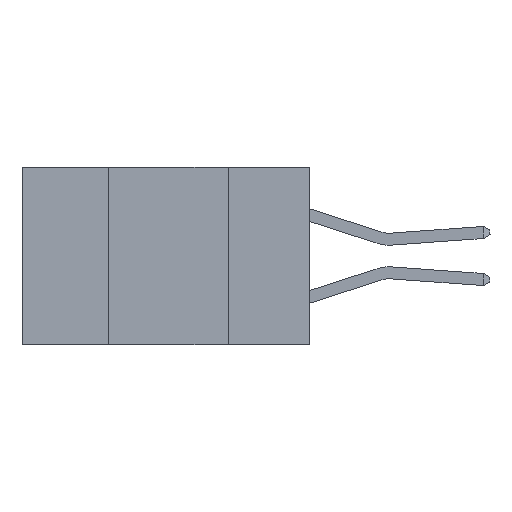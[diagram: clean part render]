
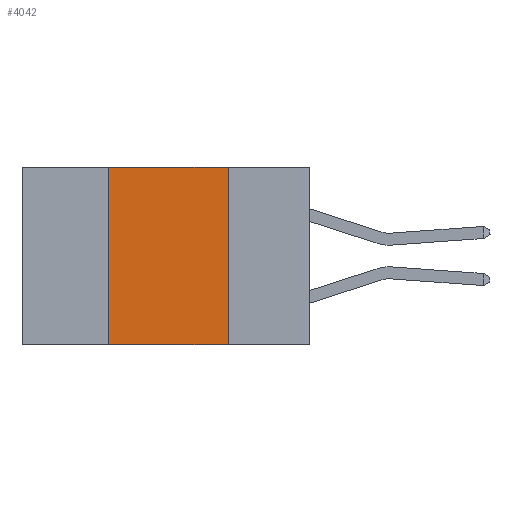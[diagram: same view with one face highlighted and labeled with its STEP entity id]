
A CAD part, left-side view. The second image highlights one B-rep face of the part: STEP entity #4042.
In plain terms, the highlighted planar face has unit normal (-1, 0, 0).
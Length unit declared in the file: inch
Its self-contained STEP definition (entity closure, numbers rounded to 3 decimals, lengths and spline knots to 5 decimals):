
#372 = EDGE_CURVE ( 'NONE', #27670, #22646, #2584, .T. ) ;
#1957 = EDGE_LOOP ( 'NONE', ( #6689, #23432, #7588, #31456 ) ) ;
#1958 = VECTOR ( 'NONE', #22943, 39.37008 ) ;
#2584 = LINE ( 'NONE', #15799, #17778 ) ;
#2964 = CARTESIAN_POINT ( 'NONE',  ( 0., 0.6, -0.37 ) ) ;
#3735 = DIRECTION ( 'NONE',  ( 1., 0., 0. ) ) ;
#4042 = ADVANCED_FACE ( 'NONE', ( #15470 ), #19031, .F. ) ;
#4496 = CARTESIAN_POINT ( 'NONE',  ( 0., 0.42, -0.37 ) ) ;
#5121 = CARTESIAN_POINT ( 'NONE',  ( 0., 0.6, 0. ) ) ;
#5539 = DIRECTION ( 'NONE',  ( 0., -1., 0. ) ) ;
#6178 = LINE ( 'NONE', #25067, #24837 ) ;
#6689 = ORIENTED_EDGE ( 'NONE', *, *, #372, .F. ) ;
#6904 = CARTESIAN_POINT ( 'NONE',  ( 0., 0.17, -0.37 ) ) ;
#7294 = EDGE_CURVE ( 'NONE', #20419, #8182, #6178, .T. ) ;
#7588 = ORIENTED_EDGE ( 'NONE', *, *, #7294, .F. ) ;
#8182 = VERTEX_POINT ( 'NONE', #10672 ) ;
#9944 = DIRECTION ( 'NONE',  ( 0., 0., 1. ) ) ;
#10672 = CARTESIAN_POINT ( 'NONE',  ( 0., 0.42, 0. ) ) ;
#12669 = AXIS2_PLACEMENT_3D ( 'NONE', #31528, #3735, #21533 ) ;
#14795 = CARTESIAN_POINT ( 'NONE',  ( 0., 0.17, 0. ) ) ;
#15470 = FACE_OUTER_BOUND ( 'NONE', #1957, .T. ) ;
#15799 = CARTESIAN_POINT ( 'NONE',  ( 0., 0.17, 0. ) ) ;
#16962 = DIRECTION ( 'NONE',  ( 0., 0., -1. ) ) ;
#17778 = VECTOR ( 'NONE', #16962, 39.37008 ) ;
#17786 = VECTOR ( 'NONE', #5539, 39.37008 ) ;
#19031 = PLANE ( 'NONE',  #12669 ) ;
#20419 = VERTEX_POINT ( 'NONE', #4496 ) ;
#21533 = DIRECTION ( 'NONE',  ( 0., 0., -1. ) ) ;
#22646 = VERTEX_POINT ( 'NONE', #6904 ) ;
#22943 = DIRECTION ( 'NONE',  ( 0., -1., 0. ) ) ;
#23432 = ORIENTED_EDGE ( 'NONE', *, *, #24104, .F. ) ;
#24104 = EDGE_CURVE ( 'NONE', #8182, #27670, #28200, .T. ) ;
#24469 = LINE ( 'NONE', #2964, #17786 ) ;
#24837 = VECTOR ( 'NONE', #9944, 39.37008 ) ;
#24930 = EDGE_CURVE ( 'NONE', #20419, #22646, #24469, .T. ) ;
#25067 = CARTESIAN_POINT ( 'NONE',  ( 0., 0.42, 0. ) ) ;
#27670 = VERTEX_POINT ( 'NONE', #14795 ) ;
#28200 = LINE ( 'NONE', #5121, #1958 ) ;
#31456 = ORIENTED_EDGE ( 'NONE', *, *, #24930, .T. ) ;
#31528 = CARTESIAN_POINT ( 'NONE',  ( 0., 0.6, 0. ) ) ;
